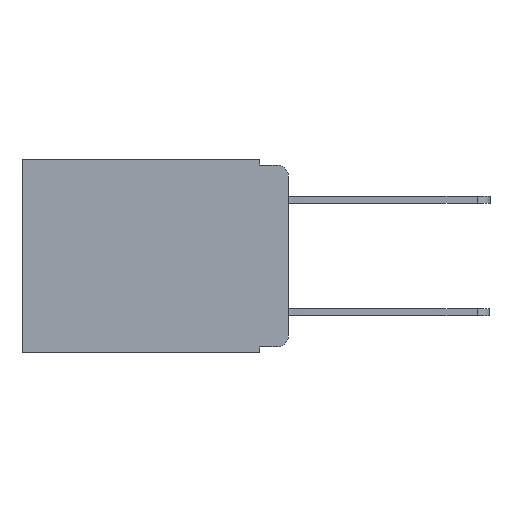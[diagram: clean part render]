
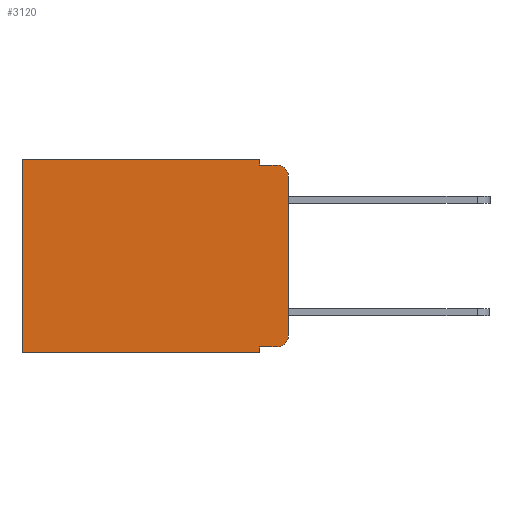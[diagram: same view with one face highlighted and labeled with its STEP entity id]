
A CAD part, left-side view. The second image highlights one B-rep face of the part: STEP entity #3120.
In plain terms, the highlighted planar face has unit normal (-1, 0, 0).
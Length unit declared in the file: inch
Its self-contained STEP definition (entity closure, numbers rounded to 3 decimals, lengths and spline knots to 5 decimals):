
#75 = CARTESIAN_POINT ( 'NONE',  ( 0.298, 0., 0. ) ) ;
#275 = ORIENTED_EDGE ( 'NONE', *, *, #2846, .F. ) ;
#486 = VERTEX_POINT ( 'NONE', #9330 ) ;
#559 = LINE ( 'NONE', #4861, #10024 ) ;
#565 = DIRECTION ( 'NONE',  ( 0., 0., -1. ) ) ;
#624 = CARTESIAN_POINT ( 'NONE',  ( 0.298, 0.051, -0.01 ) ) ;
#634 = LINE ( 'NONE', #1504, #3690 ) ;
#1138 = ORIENTED_EDGE ( 'NONE', *, *, #3007, .F. ) ;
#1283 = CARTESIAN_POINT ( 'NONE',  ( 0.298, 0., 0. ) ) ;
#1306 = VERTEX_POINT ( 'NONE', #7301 ) ;
#1504 = CARTESIAN_POINT ( 'NONE',  ( 0.298, 0.473, 0. ) ) ;
#1664 = DIRECTION ( 'NONE',  ( 0., 0., -1. ) ) ;
#1721 = CARTESIAN_POINT ( 'NONE',  ( 0.298, 0., -0.343 ) ) ;
#1818 = EDGE_LOOP ( 'NONE', ( #8002, #4267, #1138, #275, #8664, #6944, #8821, #8974, #8273, #9263 ) ) ;
#1895 = CARTESIAN_POINT ( 'NONE',  ( 0.298, 0.02, -0.333 ) ) ;
#1925 = CARTESIAN_POINT ( 'NONE',  ( 0.298, 0.02, -0.313 ) ) ;
#2102 = EDGE_CURVE ( 'NONE', #7060, #6484, #8507, .T. ) ;
#2179 = CARTESIAN_POINT ( 'NONE',  ( 0.298, 0., -0.03 ) ) ;
#2298 = LINE ( 'NONE', #7418, #4617 ) ;
#2418 = DIRECTION ( 'NONE',  ( 0., 1., 0. ) ) ;
#2469 = CIRCLE ( 'NONE', #11145, 0.02 ) ;
#2483 = VECTOR ( 'NONE', #9324, 39.37008 ) ;
#2810 = EDGE_CURVE ( 'NONE', #4870, #486, #634, .T. ) ;
#2846 = EDGE_CURVE ( 'NONE', #11394, #5177, #9649, .T. ) ;
#2994 = VECTOR ( 'NONE', #10818, 39.37008 ) ;
#3007 = EDGE_CURVE ( 'NONE', #5177, #1306, #2298, .T. ) ;
#3111 = EDGE_CURVE ( 'NONE', #3989, #1306, #2469, .T. ) ;
#3120 = ADVANCED_FACE ( 'NONE', ( #7379 ), #10828, .F. ) ;
#3141 = CARTESIAN_POINT ( 'NONE',  ( 0.298, 0.473, 0. ) ) ;
#3579 = VECTOR ( 'NONE', #3880, 39.37008 ) ;
#3690 = VECTOR ( 'NONE', #565, 39.37008 ) ;
#3880 = DIRECTION ( 'NONE',  ( 0., -1., 0. ) ) ;
#3916 = EDGE_CURVE ( 'NONE', #6484, #7503, #10164, .T. ) ;
#3989 = VERTEX_POINT ( 'NONE', #2179 ) ;
#4267 = ORIENTED_EDGE ( 'NONE', *, *, #3111, .T. ) ;
#4361 = AXIS2_PLACEMENT_3D ( 'NONE', #1283, #4451, #5414 ) ;
#4389 = VECTOR ( 'NONE', #8446, 39.37008 ) ;
#4451 = DIRECTION ( 'NONE',  ( 1., 0., 0. ) ) ;
#4585 = CARTESIAN_POINT ( 'NONE',  ( 0.298, 0.051, -0.333 ) ) ;
#4617 = VECTOR ( 'NONE', #9209, 39.37008 ) ;
#4861 = CARTESIAN_POINT ( 'NONE',  ( 0.298, 0., 0. ) ) ;
#4870 = VERTEX_POINT ( 'NONE', #3141 ) ;
#4966 = EDGE_CURVE ( 'NONE', #11394, #4870, #559, .T. ) ;
#5177 = VERTEX_POINT ( 'NONE', #624 ) ;
#5414 = DIRECTION ( 'NONE',  ( 0., 0., -1. ) ) ;
#5867 = EDGE_CURVE ( 'NONE', #7060, #8564, #10232, .T. ) ;
#5930 = EDGE_CURVE ( 'NONE', #3989, #7503, #9141, .T. ) ;
#6391 = EDGE_CURVE ( 'NONE', #8564, #486, #9992, .T. ) ;
#6484 = VERTEX_POINT ( 'NONE', #1895 ) ;
#6944 = ORIENTED_EDGE ( 'NONE', *, *, #2810, .T. ) ;
#7060 = VERTEX_POINT ( 'NONE', #8250 ) ;
#7301 = CARTESIAN_POINT ( 'NONE',  ( 0.298, 0.02, -0.01 ) ) ;
#7379 = FACE_OUTER_BOUND ( 'NONE', #1818, .T. ) ;
#7418 = CARTESIAN_POINT ( 'NONE',  ( 0.298, 0.051, -0.01 ) ) ;
#7503 = VERTEX_POINT ( 'NONE', #7689 ) ;
#7689 = CARTESIAN_POINT ( 'NONE',  ( 0.298, 0., -0.313 ) ) ;
#8002 = ORIENTED_EDGE ( 'NONE', *, *, #5930, .F. ) ;
#8049 = VECTOR ( 'NONE', #1664, 39.37008 ) ;
#8053 = AXIS2_PLACEMENT_3D ( 'NONE', #1925, #10830, #10819 ) ;
#8250 = CARTESIAN_POINT ( 'NONE',  ( 0.298, 0.051, -0.333 ) ) ;
#8273 = ORIENTED_EDGE ( 'NONE', *, *, #2102, .T. ) ;
#8446 = DIRECTION ( 'NONE',  ( 0., 0., -1. ) ) ;
#8497 = DIRECTION ( 'NONE',  ( -1., 0., 0. ) ) ;
#8507 = LINE ( 'NONE', #4585, #3579 ) ;
#8564 = VERTEX_POINT ( 'NONE', #10101 ) ;
#8664 = ORIENTED_EDGE ( 'NONE', *, *, #4966, .T. ) ;
#8821 = ORIENTED_EDGE ( 'NONE', *, *, #6391, .F. ) ;
#8974 = ORIENTED_EDGE ( 'NONE', *, *, #5867, .F. ) ;
#9141 = LINE ( 'NONE', #75, #4389 ) ;
#9209 = DIRECTION ( 'NONE',  ( 0., -1., 0. ) ) ;
#9263 = ORIENTED_EDGE ( 'NONE', *, *, #3916, .T. ) ;
#9324 = DIRECTION ( 'NONE',  ( 0., 0., -1. ) ) ;
#9330 = CARTESIAN_POINT ( 'NONE',  ( 0.298, 0.473, -0.343 ) ) ;
#9649 = LINE ( 'NONE', #9984, #2483 ) ;
#9960 = CARTESIAN_POINT ( 'NONE',  ( 0.298, 0.051, 0. ) ) ;
#9984 = CARTESIAN_POINT ( 'NONE',  ( 0.298, 0.051, 0. ) ) ;
#9992 = LINE ( 'NONE', #1721, #2994 ) ;
#10024 = VECTOR ( 'NONE', #2418, 39.37008 ) ;
#10101 = CARTESIAN_POINT ( 'NONE',  ( 0.298, 0.051, -0.343 ) ) ;
#10164 = CIRCLE ( 'NONE', #8053, 0.02 ) ;
#10232 = LINE ( 'NONE', #11441, #8049 ) ;
#10301 = DIRECTION ( 'NONE',  ( 0., 0., -1. ) ) ;
#10818 = DIRECTION ( 'NONE',  ( 0., 1., 0. ) ) ;
#10819 = DIRECTION ( 'NONE',  ( 0., 0., -1. ) ) ;
#10828 = PLANE ( 'NONE',  #4361 ) ;
#10830 = DIRECTION ( 'NONE',  ( -1., 0., 0. ) ) ;
#11137 = CARTESIAN_POINT ( 'NONE',  ( 0.298, 0.02, -0.03 ) ) ;
#11145 = AXIS2_PLACEMENT_3D ( 'NONE', #11137, #8497, #10301 ) ;
#11394 = VERTEX_POINT ( 'NONE', #9960 ) ;
#11441 = CARTESIAN_POINT ( 'NONE',  ( 0.298, 0.051, 0. ) ) ;
